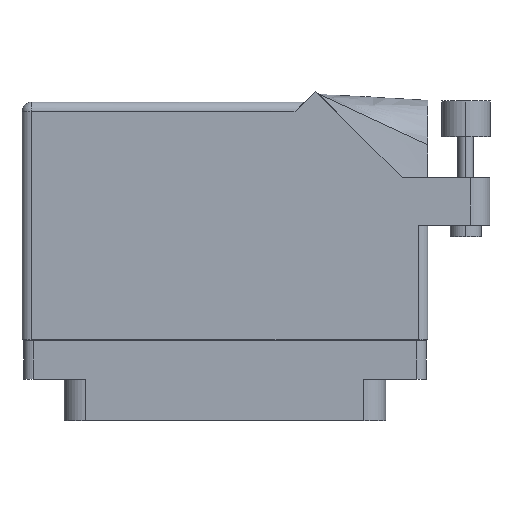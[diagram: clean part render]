
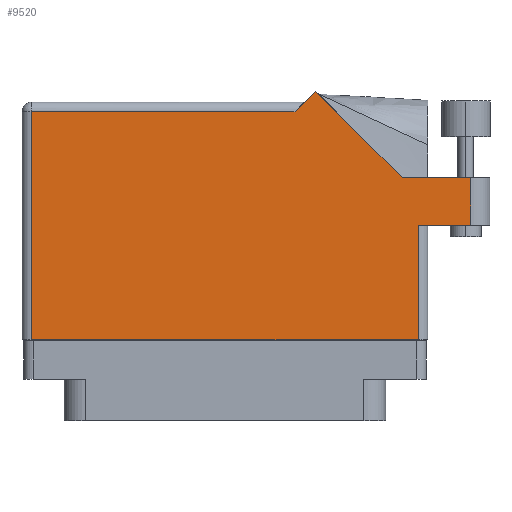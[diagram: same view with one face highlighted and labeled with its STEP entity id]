
A CAD part, front view. The second image highlights one B-rep face of the part: STEP entity #9520.
In plain terms, the highlighted face is planar.
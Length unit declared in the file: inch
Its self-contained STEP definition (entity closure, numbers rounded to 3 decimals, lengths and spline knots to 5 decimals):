
#1920 = VERTEX_POINT ( 'NONE', #47654 ) ;
#2225 = VERTEX_POINT ( 'NONE', #33233 ) ;
#2652 = CARTESIAN_POINT ( 'NONE',  ( 1.706, 0.944, 0.455 ) ) ;
#2823 = DIRECTION ( 'NONE',  ( -1., 0., 0. ) ) ;
#3487 = LINE ( 'NONE', #36037, #33605 ) ;
#3521 = DIRECTION ( 'NONE',  ( 0., -1., 0. ) ) ;
#5464 = EDGE_LOOP ( 'NONE', ( #25104, #36047, #47238, #30240, #13689, #17309, #28030, #34493, #39848 ) ) ;
#5572 = VERTEX_POINT ( 'NONE', #46478 ) ;
#6667 = DIRECTION ( 'NONE',  ( -1., 0., 0. ) ) ;
#6737 = CARTESIAN_POINT ( 'NONE',  ( -1.306, 1.43, 0.455 ) ) ;
#9520 = ADVANCED_FACE ( 'NONE', ( #31482 ), #47202, .F. ) ;
#11287 = VERTEX_POINT ( 'NONE', #34769 ) ;
#11503 = EDGE_CURVE ( 'NONE', #32689, #2225, #3487, .T. ) ;
#12091 = VERTEX_POINT ( 'NONE', #42555 ) ;
#13551 = CARTESIAN_POINT ( 'NONE',  ( 1.581, 0.637, 0.455 ) ) ;
#13689 = ORIENTED_EDGE ( 'NONE', *, *, #46046, .T. ) ;
#13912 = AXIS2_PLACEMENT_3D ( 'NONE', #6737, #47035, #25157 ) ;
#14873 = CARTESIAN_POINT ( 'NONE',  ( 1.244, 0.637, 0.455 ) ) ;
#15445 = VECTOR ( 'NONE', #22056, 39.37008 ) ;
#15738 = DIRECTION ( 'NONE',  ( 1., 0., 0. ) ) ;
#17309 = ORIENTED_EDGE ( 'NONE', *, *, #22604, .T. ) ;
#17566 = EDGE_CURVE ( 'NONE', #1920, #32689, #40940, .T. ) ;
#17632 = EDGE_CURVE ( 'NONE', #2225, #5572, #17778, .T. ) ;
#17778 = LINE ( 'NONE', #2652, #31104 ) ;
#18897 = EDGE_CURVE ( 'NONE', #42082, #1920, #34907, .T. ) ;
#18958 = VERTEX_POINT ( 'NONE', #40605 ) ;
#19664 = LINE ( 'NONE', #45421, #21998 ) ;
#20593 = LINE ( 'NONE', #32437, #36259 ) ;
#20602 = VECTOR ( 'NONE', #32749, 39.37008 ) ;
#21401 = CARTESIAN_POINT ( 'NONE',  ( 0.513, 1.43, 0.455 ) ) ;
#21833 = CARTESIAN_POINT ( 'NONE',  ( 1.244, -0.1, 0.455 ) ) ;
#21998 = VECTOR ( 'NONE', #3521, 39.37008 ) ;
#22056 = DIRECTION ( 'NONE',  ( 1., 0., 0. ) ) ;
#22604 = EDGE_CURVE ( 'NONE', #18958, #11287, #20593, .T. ) ;
#23124 = CARTESIAN_POINT ( 'NONE',  ( -1.244, -0.1, 0.455 ) ) ;
#24054 = LINE ( 'NONE', #21401, #20602 ) ;
#24958 = VERTEX_POINT ( 'NONE', #23124 ) ;
#25104 = ORIENTED_EDGE ( 'NONE', *, *, #17566, .T. ) ;
#25157 = DIRECTION ( 'NONE',  ( -1., 0., 0. ) ) ;
#26158 = DIRECTION ( 'NONE',  ( 0., 1., 0. ) ) ;
#27433 = LINE ( 'NONE', #41628, #45987 ) ;
#27438 = DIRECTION ( 'NONE',  ( -0.707, 0.707, 0. ) ) ;
#28030 = ORIENTED_EDGE ( 'NONE', *, *, #33285, .T. ) ;
#28432 = LINE ( 'NONE', #38662, #34279 ) ;
#30240 = ORIENTED_EDGE ( 'NONE', *, *, #38034, .T. ) ;
#31104 = VECTOR ( 'NONE', #2823, 39.37008 ) ;
#31482 = FACE_OUTER_BOUND ( 'NONE', #5464, .T. ) ;
#32437 = CARTESIAN_POINT ( 'NONE',  ( -1.306, 1.368, 0.455 ) ) ;
#32689 = VERTEX_POINT ( 'NONE', #13551 ) ;
#32749 = DIRECTION ( 'NONE',  ( -0.707, -0.707, 0. ) ) ;
#33233 = CARTESIAN_POINT ( 'NONE',  ( 1.581, 0.944, 0.455 ) ) ;
#33285 = EDGE_CURVE ( 'NONE', #11287, #24958, #19664, .T. ) ;
#33605 = VECTOR ( 'NONE', #36538, 39.37008 ) ;
#34279 = VECTOR ( 'NONE', #27438, 39.37008 ) ;
#34493 = ORIENTED_EDGE ( 'NONE', *, *, #46701, .T. ) ;
#34769 = CARTESIAN_POINT ( 'NONE',  ( -1.244, 1.368, 0.455 ) ) ;
#34907 = LINE ( 'NONE', #14873, #38375 ) ;
#36037 = CARTESIAN_POINT ( 'NONE',  ( 1.581, 0.944, 0.455 ) ) ;
#36047 = ORIENTED_EDGE ( 'NONE', *, *, #11503, .T. ) ;
#36259 = VECTOR ( 'NONE', #6667, 39.37008 ) ;
#36538 = DIRECTION ( 'NONE',  ( 0., 1., 0. ) ) ;
#38034 = EDGE_CURVE ( 'NONE', #5572, #12091, #28432, .T. ) ;
#38375 = VECTOR ( 'NONE', #26158, 39.37008 ) ;
#38662 = CARTESIAN_POINT ( 'NONE',  ( 1.14042, 0.944, 0.455 ) ) ;
#39848 = ORIENTED_EDGE ( 'NONE', *, *, #18897, .T. ) ;
#40503 = CARTESIAN_POINT ( 'NONE',  ( 1.306, 0.637, 0.455 ) ) ;
#40605 = CARTESIAN_POINT ( 'NONE',  ( 0.451, 1.368, 0.455 ) ) ;
#40940 = LINE ( 'NONE', #40503, #15445 ) ;
#41628 = CARTESIAN_POINT ( 'NONE',  ( -1.306, -0.1, 0.455 ) ) ;
#42082 = VERTEX_POINT ( 'NONE', #21833 ) ;
#42555 = CARTESIAN_POINT ( 'NONE',  ( 0.58371, 1.50071, 0.455 ) ) ;
#45421 = CARTESIAN_POINT ( 'NONE',  ( -1.244, -0.1, 0.455 ) ) ;
#45987 = VECTOR ( 'NONE', #15738, 39.37008 ) ;
#46046 = EDGE_CURVE ( 'NONE', #12091, #18958, #24054, .T. ) ;
#46478 = CARTESIAN_POINT ( 'NONE',  ( 1.14042, 0.944, 0.455 ) ) ;
#46701 = EDGE_CURVE ( 'NONE', #24958, #42082, #27433, .T. ) ;
#47035 = DIRECTION ( 'NONE',  ( 0., 0., -1. ) ) ;
#47202 = PLANE ( 'NONE',  #13912 ) ;
#47238 = ORIENTED_EDGE ( 'NONE', *, *, #17632, .T. ) ;
#47654 = CARTESIAN_POINT ( 'NONE',  ( 1.244, 0.637, 0.455 ) ) ;
